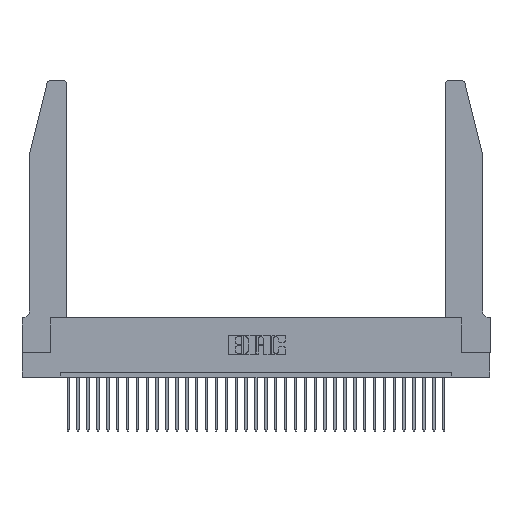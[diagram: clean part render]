
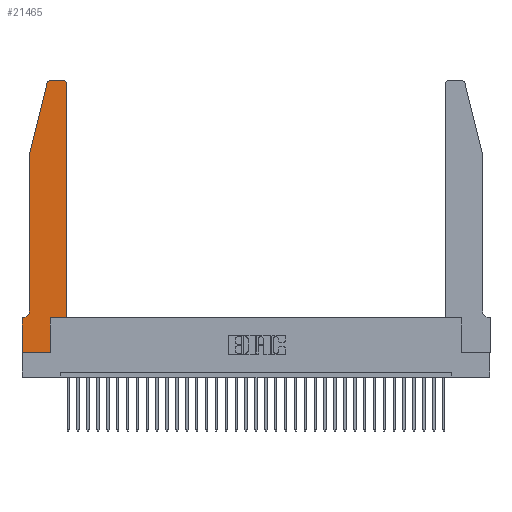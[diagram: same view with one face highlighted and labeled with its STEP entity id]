
A CAD part, top view. The second image highlights one B-rep face of the part: STEP entity #21465.
In plain terms, the highlighted planar face has unit normal (0, 0, 1).
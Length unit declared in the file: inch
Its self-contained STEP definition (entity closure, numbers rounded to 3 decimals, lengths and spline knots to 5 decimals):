
#343 = CIRCLE ( 'NONE', #29497, 0.07 ) ;
#454 = LINE ( 'NONE', #10525, #31380 ) ;
#924 = CARTESIAN_POINT ( 'NONE',  ( 0., 0.35, 0.37 ) ) ;
#944 = EDGE_CURVE ( 'NONE', #15280, #18709, #13337, .T. ) ;
#993 = DIRECTION ( 'NONE',  ( 1., 0., 0. ) ) ;
#1190 = VECTOR ( 'NONE', #24892, 39.37008 ) ;
#1624 = EDGE_LOOP ( 'NONE', ( #33340, #3875, #8495, #25899, #17633, #12726, #33712, #4137, #31598, #8306, #8927, #22832 ) ) ;
#1768 = CARTESIAN_POINT ( 'NONE',  ( 0.0055, 0.35, 0.37 ) ) ;
#2055 = CARTESIAN_POINT ( 'NONE',  ( 0.4505, 0.35, 0.37 ) ) ;
#2252 = CARTESIAN_POINT ( 'NONE',  ( 0., 0.35, 0.37 ) ) ;
#2623 = LINE ( 'NONE', #24542, #22635 ) ;
#2645 = AXIS2_PLACEMENT_3D ( 'NONE', #2252, #23988, #16310 ) ;
#2836 = VECTOR ( 'NONE', #33879, 39.37008 ) ;
#3296 = FACE_OUTER_BOUND ( 'NONE', #1624, .T. ) ;
#3793 = CIRCLE ( 'NONE', #15154, 0.03 ) ;
#3875 = ORIENTED_EDGE ( 'NONE', *, *, #5421, .T. ) ;
#4137 = ORIENTED_EDGE ( 'NONE', *, *, #23787, .T. ) ;
#4237 = DIRECTION ( 'NONE',  ( 1., 0., 0. ) ) ;
#4557 = DIRECTION ( 'NONE',  ( 1., 0., 0. ) ) ;
#5421 = EDGE_CURVE ( 'NONE', #16689, #13315, #3793, .T. ) ;
#6044 = VECTOR ( 'NONE', #993, 39.37008 ) ;
#6782 = CARTESIAN_POINT ( 'NONE',  ( 0.284, 2.72, 0.37 ) ) ;
#8152 = LINE ( 'NONE', #29681, #6044 ) ;
#8306 = ORIENTED_EDGE ( 'NONE', *, *, #31843, .T. ) ;
#8495 = ORIENTED_EDGE ( 'NONE', *, *, #14162, .T. ) ;
#8641 = CARTESIAN_POINT ( 'NONE',  ( 0.0055, 0.42, 0.37 ) ) ;
#8927 = ORIENTED_EDGE ( 'NONE', *, *, #18425, .T. ) ;
#9672 = CARTESIAN_POINT ( 'NONE',  ( 0., 0., 0.37 ) ) ;
#9678 = DIRECTION ( 'NONE',  ( 0., 0., 1. ) ) ;
#9712 = CARTESIAN_POINT ( 'NONE',  ( 0.0755, 0.35, 0.37 ) ) ;
#10040 = VERTEX_POINT ( 'NONE', #924 ) ;
#10525 = CARTESIAN_POINT ( 'NONE',  ( 0.0755, 2., 0.37 ) ) ;
#10659 = VECTOR ( 'NONE', #12899, 39.37008 ) ;
#10796 = EDGE_CURVE ( 'NONE', #16036, #17907, #343, .T. ) ;
#12280 = DIRECTION ( 'NONE',  ( 0., -1., 0. ) ) ;
#12726 = ORIENTED_EDGE ( 'NONE', *, *, #14402, .T. ) ;
#12875 = VECTOR ( 'NONE', #18561, 39.37008 ) ;
#12899 = DIRECTION ( 'NONE',  ( 0., 1., 0. ) ) ;
#13315 = VERTEX_POINT ( 'NONE', #19226 ) ;
#13337 = LINE ( 'NONE', #28895, #1190 ) ;
#13678 = AXIS2_PLACEMENT_3D ( 'NONE', #30119, #33524, #4237 ) ;
#14162 = EDGE_CURVE ( 'NONE', #13315, #25208, #454, .T. ) ;
#14175 = CARTESIAN_POINT ( 'NONE',  ( 0.4505, 2.72, 0.37 ) ) ;
#14402 = EDGE_CURVE ( 'NONE', #17907, #10040, #29306, .T. ) ;
#14528 = LINE ( 'NONE', #26488, #12875 ) ;
#15154 = AXIS2_PLACEMENT_3D ( 'NONE', #6782, #9678, #4557 ) ;
#15259 = CARTESIAN_POINT ( 'NONE',  ( 0., 0., 0.37 ) ) ;
#15280 = VERTEX_POINT ( 'NONE', #31116 ) ;
#15413 = LINE ( 'NONE', #15259, #2836 ) ;
#15846 = DIRECTION ( 'NONE',  ( -0.239, -0.971, 0. ) ) ;
#16036 = VERTEX_POINT ( 'NONE', #24839 ) ;
#16310 = DIRECTION ( 'NONE',  ( 1., 0., 0. ) ) ;
#16525 = PLANE ( 'NONE',  #2645 ) ;
#16689 = VERTEX_POINT ( 'NONE', #33787 ) ;
#17633 = ORIENTED_EDGE ( 'NONE', *, *, #10796, .T. ) ;
#17907 = VERTEX_POINT ( 'NONE', #1768 ) ;
#18425 = EDGE_CURVE ( 'NONE', #25652, #23644, #29844, .T. ) ;
#18543 = VERTEX_POINT ( 'NONE', #30434 ) ;
#18561 = DIRECTION ( 'NONE',  ( 1., 0., 0. ) ) ;
#18709 = VERTEX_POINT ( 'NONE', #20728 ) ;
#18854 = DIRECTION ( 'NONE',  ( -1., 0., 0. ) ) ;
#19226 = CARTESIAN_POINT ( 'NONE',  ( 0.25487, 2.72718, 0.37 ) ) ;
#20488 = CARTESIAN_POINT ( 'NONE',  ( 0.0755, 2., 0.37 ) ) ;
#20602 = DIRECTION ( 'NONE',  ( -1., 0., 0. ) ) ;
#20728 = CARTESIAN_POINT ( 'NONE',  ( 0.2865, 0.35, 0.37 ) ) ;
#21465 = ADVANCED_FACE ( 'NONE', ( #3296 ), #16525, .T. ) ;
#22130 = EDGE_CURVE ( 'NONE', #10040, #25112, #15413, .T. ) ;
#22226 = VECTOR ( 'NONE', #20602, 39.37008 ) ;
#22635 = VECTOR ( 'NONE', #18854, 39.37008 ) ;
#22832 = ORIENTED_EDGE ( 'NONE', *, *, #25954, .T. ) ;
#23644 = VERTEX_POINT ( 'NONE', #14175 ) ;
#23787 = EDGE_CURVE ( 'NONE', #25112, #15280, #8152, .T. ) ;
#23988 = DIRECTION ( 'NONE',  ( 0., 0., 1. ) ) ;
#24542 = CARTESIAN_POINT ( 'NONE',  ( 0.2605, 2.75, 0.37 ) ) ;
#24839 = CARTESIAN_POINT ( 'NONE',  ( 0.0755, 0.42, 0.37 ) ) ;
#24892 = DIRECTION ( 'NONE',  ( 0., 1., 0. ) ) ;
#25112 = VERTEX_POINT ( 'NONE', #9672 ) ;
#25208 = VERTEX_POINT ( 'NONE', #20488 ) ;
#25375 = LINE ( 'NONE', #28122, #28725 ) ;
#25652 = VERTEX_POINT ( 'NONE', #32166 ) ;
#25899 = ORIENTED_EDGE ( 'NONE', *, *, #32923, .T. ) ;
#25954 = EDGE_CURVE ( 'NONE', #23644, #18543, #26375, .T. ) ;
#26375 = CIRCLE ( 'NONE', #13678, 0.03 ) ;
#26488 = CARTESIAN_POINT ( 'NONE',  ( 0.4505, 0.35, 0.37 ) ) ;
#27266 = DIRECTION ( 'NONE',  ( -1., 0., 0. ) ) ;
#27605 = DIRECTION ( 'NONE',  ( 0., 0., -1. ) ) ;
#28122 = CARTESIAN_POINT ( 'NONE',  ( 0.0755, 2., 0.37 ) ) ;
#28725 = VECTOR ( 'NONE', #12280, 39.37008 ) ;
#28895 = CARTESIAN_POINT ( 'NONE',  ( 0.2865, 0.35, 0.37 ) ) ;
#29306 = LINE ( 'NONE', #9712, #22226 ) ;
#29497 = AXIS2_PLACEMENT_3D ( 'NONE', #8641, #27605, #27266 ) ;
#29681 = CARTESIAN_POINT ( 'NONE',  ( 0., 0., 0.37 ) ) ;
#29844 = LINE ( 'NONE', #2055, #10659 ) ;
#30119 = CARTESIAN_POINT ( 'NONE',  ( 0.4205, 2.72, 0.37 ) ) ;
#30434 = CARTESIAN_POINT ( 'NONE',  ( 0.4205, 2.75, 0.37 ) ) ;
#31116 = CARTESIAN_POINT ( 'NONE',  ( 0.2865, 0., 0.37 ) ) ;
#31380 = VECTOR ( 'NONE', #15846, 39.37008 ) ;
#31598 = ORIENTED_EDGE ( 'NONE', *, *, #944, .T. ) ;
#31843 = EDGE_CURVE ( 'NONE', #18709, #25652, #14528, .T. ) ;
#32166 = CARTESIAN_POINT ( 'NONE',  ( 0.4505, 0.35, 0.37 ) ) ;
#32662 = EDGE_CURVE ( 'NONE', #18543, #16689, #2623, .T. ) ;
#32923 = EDGE_CURVE ( 'NONE', #25208, #16036, #25375, .T. ) ;
#33340 = ORIENTED_EDGE ( 'NONE', *, *, #32662, .T. ) ;
#33524 = DIRECTION ( 'NONE',  ( 0., 0., 1. ) ) ;
#33712 = ORIENTED_EDGE ( 'NONE', *, *, #22130, .T. ) ;
#33787 = CARTESIAN_POINT ( 'NONE',  ( 0.284, 2.75, 0.37 ) ) ;
#33879 = DIRECTION ( 'NONE',  ( 0., -1., 0. ) ) ;
